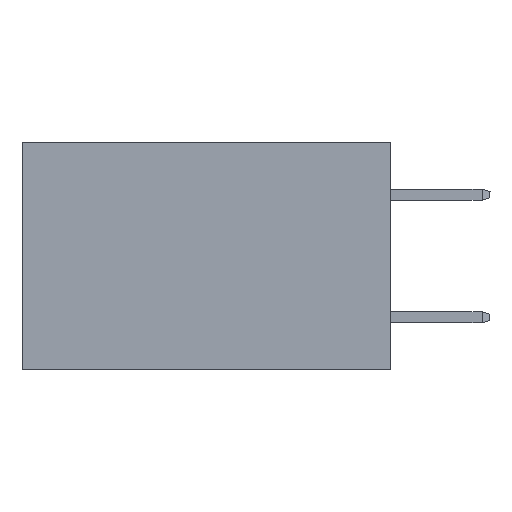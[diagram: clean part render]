
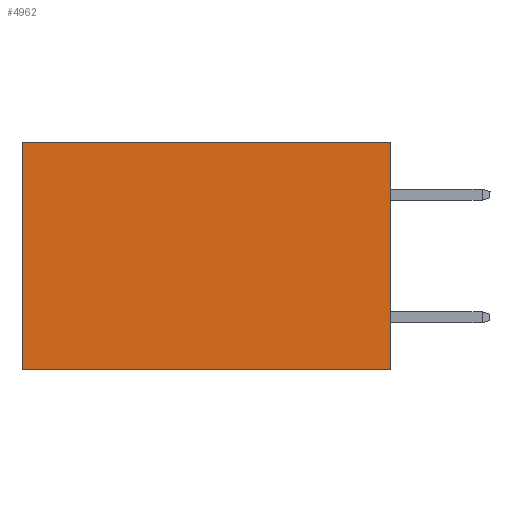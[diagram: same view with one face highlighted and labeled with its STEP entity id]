
A CAD part, left-side view. The second image highlights one B-rep face of the part: STEP entity #4962.
In plain terms, the highlighted planar face has unit normal (-1, 0, 0).
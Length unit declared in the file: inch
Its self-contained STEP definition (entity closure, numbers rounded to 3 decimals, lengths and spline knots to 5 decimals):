
#151 = ORIENTED_EDGE ( 'NONE', *, *, #8705, .F. ) ;
#560 = DIRECTION ( 'NONE',  ( 0., 1., 0. ) ) ;
#745 = LINE ( 'NONE', #893, #6423 ) ;
#893 = CARTESIAN_POINT ( 'NONE',  ( 0.2875, 0., 0. ) ) ;
#960 = ORIENTED_EDGE ( 'NONE', *, *, #1790, .T. ) ;
#1030 = CARTESIAN_POINT ( 'NONE',  ( 0.2875, 0., 0. ) ) ;
#1756 = PLANE ( 'NONE',  #7563 ) ;
#1790 = EDGE_CURVE ( 'NONE', #1881, #3912, #5958, .T. ) ;
#1870 = ORIENTED_EDGE ( 'NONE', *, *, #5289, .F. ) ;
#1881 = VERTEX_POINT ( 'NONE', #7161 ) ;
#2147 = VERTEX_POINT ( 'NONE', #3562 ) ;
#2162 = FACE_OUTER_BOUND ( 'NONE', #5560, .T. ) ;
#3129 = LINE ( 'NONE', #4580, #3868 ) ;
#3205 = DIRECTION ( 'NONE',  ( 0., 0., -1. ) ) ;
#3562 = CARTESIAN_POINT ( 'NONE',  ( 0.2875, 0.6, -0.37 ) ) ;
#3741 = DIRECTION ( 'NONE',  ( 1., 0., 0. ) ) ;
#3868 = VECTOR ( 'NONE', #560, 39.37008 ) ;
#3912 = VERTEX_POINT ( 'NONE', #8307 ) ;
#4370 = VERTEX_POINT ( 'NONE', #8153 ) ;
#4580 = CARTESIAN_POINT ( 'NONE',  ( 0.2875, 0., -0.37 ) ) ;
#4962 = ADVANCED_FACE ( 'NONE', ( #2162 ), #1756, .F. ) ;
#5023 = ORIENTED_EDGE ( 'NONE', *, *, #5089, .T. ) ;
#5089 = EDGE_CURVE ( 'NONE', #3912, #2147, #7678, .T. ) ;
#5289 = EDGE_CURVE ( 'NONE', #1881, #4370, #745, .T. ) ;
#5560 = EDGE_LOOP ( 'NONE', ( #5023, #151, #1870, #960 ) ) ;
#5715 = DIRECTION ( 'NONE',  ( 0., 1., 0. ) ) ;
#5958 = LINE ( 'NONE', #1030, #6268 ) ;
#6268 = VECTOR ( 'NONE', #5715, 39.37008 ) ;
#6423 = VECTOR ( 'NONE', #6990, 39.37008 ) ;
#6503 = DIRECTION ( 'NONE',  ( 0., 0., -1. ) ) ;
#6603 = CARTESIAN_POINT ( 'NONE',  ( 0.2875, 0.6, 0. ) ) ;
#6990 = DIRECTION ( 'NONE',  ( 0., 0., -1. ) ) ;
#7145 = CARTESIAN_POINT ( 'NONE',  ( 0.2875, 0., 0. ) ) ;
#7161 = CARTESIAN_POINT ( 'NONE',  ( 0.2875, 0., 0. ) ) ;
#7563 = AXIS2_PLACEMENT_3D ( 'NONE', #7145, #3741, #6503 ) ;
#7678 = LINE ( 'NONE', #6603, #8429 ) ;
#8153 = CARTESIAN_POINT ( 'NONE',  ( 0.2875, 0., -0.37 ) ) ;
#8307 = CARTESIAN_POINT ( 'NONE',  ( 0.2875, 0.6, 0. ) ) ;
#8429 = VECTOR ( 'NONE', #3205, 39.37008 ) ;
#8705 = EDGE_CURVE ( 'NONE', #4370, #2147, #3129, .T. ) ;
